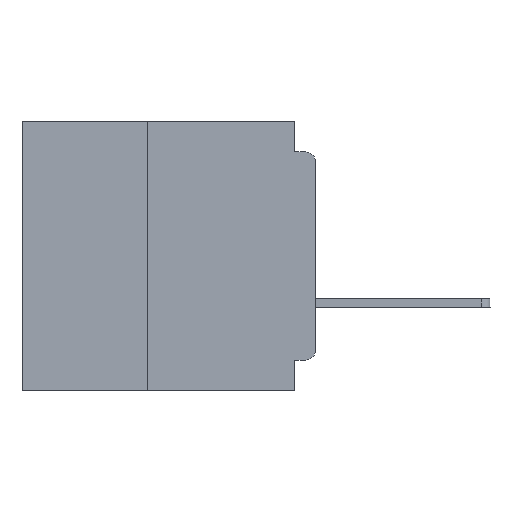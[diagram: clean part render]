
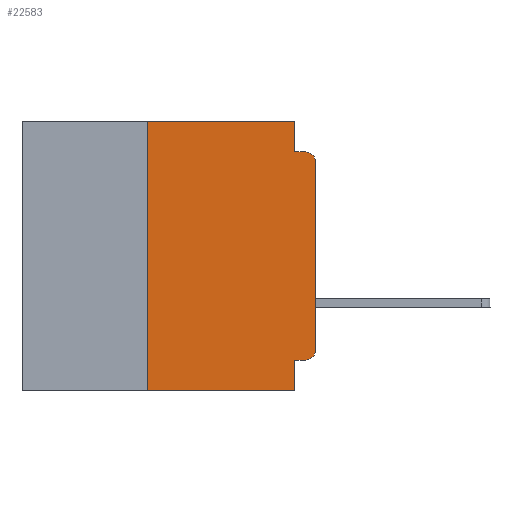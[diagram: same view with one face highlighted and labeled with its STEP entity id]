
A CAD part, left-side view. The second image highlights one B-rep face of the part: STEP entity #22583.
In plain terms, the highlighted planar face has unit normal (-1, 0, 0).
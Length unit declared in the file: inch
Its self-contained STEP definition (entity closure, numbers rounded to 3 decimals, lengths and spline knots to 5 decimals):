
#643 = ORIENTED_EDGE ( 'NONE', *, *, #54215, .T. ) ;
#1542 = DIRECTION ( 'NONE',  ( -1., 0., 0. ) ) ;
#1597 = ORIENTED_EDGE ( 'NONE', *, *, #41846, .F. ) ;
#3135 = VERTEX_POINT ( 'NONE', #16661 ) ;
#4061 = ORIENTED_EDGE ( 'NONE', *, *, #28307, .F. ) ;
#5367 = VECTOR ( 'NONE', #54887, 39.37008 ) ;
#5471 = VERTEX_POINT ( 'NONE', #65578 ) ;
#5751 = CARTESIAN_POINT ( 'NONE',  ( 0., 0.437, -0.4 ) ) ;
#8550 = EDGE_CURVE ( 'NONE', #5471, #65223, #45834, .T. ) ;
#8816 = LINE ( 'NONE', #59052, #59997 ) ;
#8886 = EDGE_CURVE ( 'NONE', #30488, #39142, #62537, .T. ) ;
#12045 = AXIS2_PLACEMENT_3D ( 'NONE', #50306, #45377, #14677 ) ;
#13266 = ORIENTED_EDGE ( 'NONE', *, *, #8550, .F. ) ;
#13970 = CARTESIAN_POINT ( 'NONE',  ( 0., 0.031, 0. ) ) ;
#14677 = DIRECTION ( 'NONE',  ( 0., 0., -1. ) ) ;
#14919 = FACE_OUTER_BOUND ( 'NONE', #15027, .T. ) ;
#15027 = EDGE_LOOP ( 'NONE', ( #643, #23600, #38655, #44543, #13266, #1597, #65956, #4061, #31773, #32027 ) ) ;
#16199 = CARTESIAN_POINT ( 'NONE',  ( 0., 0.015, -0.355 ) ) ;
#16441 = DIRECTION ( 'NONE',  ( -1., 0., 0. ) ) ;
#16661 = CARTESIAN_POINT ( 'NONE',  ( 0., 0.031, -0.4 ) ) ;
#18741 = AXIS2_PLACEMENT_3D ( 'NONE', #32315, #1542, #37465 ) ;
#18847 = AXIS2_PLACEMENT_3D ( 'NONE', #47138, #16441, #52256 ) ;
#20022 = CARTESIAN_POINT ( 'NONE',  ( 0., 0.25, -0.4 ) ) ;
#20144 = VECTOR ( 'NONE', #25814, 39.37008 ) ;
#20293 = CARTESIAN_POINT ( 'NONE',  ( 0., 0., 0. ) ) ;
#21737 = CARTESIAN_POINT ( 'NONE',  ( 0., 0.031, -0.045 ) ) ;
#22583 = ADVANCED_FACE ( 'NONE', ( #14919 ), #55152, .F. ) ;
#23600 = ORIENTED_EDGE ( 'NONE', *, *, #44344, .T. ) ;
#23817 = DIRECTION ( 'NONE',  ( 0., -1., 0. ) ) ;
#24776 = CARTESIAN_POINT ( 'NONE',  ( 0., 0., -0.355 ) ) ;
#25814 = DIRECTION ( 'NONE',  ( 0., 0., 1. ) ) ;
#28307 = EDGE_CURVE ( 'NONE', #39142, #3135, #32736, .T. ) ;
#30488 = VERTEX_POINT ( 'NONE', #16199 ) ;
#31773 = ORIENTED_EDGE ( 'NONE', *, *, #8886, .F. ) ;
#32027 = ORIENTED_EDGE ( 'NONE', *, *, #36684, .T. ) ;
#32076 = VECTOR ( 'NONE', #50921, 39.37008 ) ;
#32277 = EDGE_CURVE ( 'NONE', #51204, #55863, #8816, .T. ) ;
#32286 = VECTOR ( 'NONE', #57796, 39.37008 ) ;
#32315 = CARTESIAN_POINT ( 'NONE',  ( 0., 0.015, -0.06 ) ) ;
#32736 = LINE ( 'NONE', #62502, #58170 ) ;
#35287 = CARTESIAN_POINT ( 'NONE',  ( 0., 0.015, -0.045 ) ) ;
#36516 = LINE ( 'NONE', #5751, #63602 ) ;
#36539 = DIRECTION ( 'NONE',  ( 0., -1., 0. ) ) ;
#36684 = EDGE_CURVE ( 'NONE', #30488, #66147, #38762, .T. ) ;
#37465 = DIRECTION ( 'NONE',  ( 0., 0., -1. ) ) ;
#38655 = ORIENTED_EDGE ( 'NONE', *, *, #32277, .F. ) ;
#38762 = CIRCLE ( 'NONE', #18847, 0.015 ) ;
#39142 = VERTEX_POINT ( 'NONE', #43019 ) ;
#41498 = VERTEX_POINT ( 'NONE', #53520 ) ;
#41846 = EDGE_CURVE ( 'NONE', #47690, #5471, #45749, .T. ) ;
#43019 = CARTESIAN_POINT ( 'NONE',  ( 0., 0.031, -0.355 ) ) ;
#44344 = EDGE_CURVE ( 'NONE', #41498, #55863, #62130, .T. ) ;
#44543 = ORIENTED_EDGE ( 'NONE', *, *, #55248, .F. ) ;
#45377 = DIRECTION ( 'NONE',  ( 1., 0., 0. ) ) ;
#45749 = LINE ( 'NONE', #56334, #20144 ) ;
#45834 = LINE ( 'NONE', #47608, #32286 ) ;
#46270 = LINE ( 'NONE', #13970, #5367 ) ;
#47138 = CARTESIAN_POINT ( 'NONE',  ( 0., 0.015, -0.34 ) ) ;
#47608 = CARTESIAN_POINT ( 'NONE',  ( 0., 0.437, 0. ) ) ;
#47690 = VERTEX_POINT ( 'NONE', #20022 ) ;
#49012 = VECTOR ( 'NONE', #55296, 39.37008 ) ;
#50306 = CARTESIAN_POINT ( 'NONE',  ( 0., 0.437, 0. ) ) ;
#50921 = DIRECTION ( 'NONE',  ( 0., 0., 1. ) ) ;
#51204 = VERTEX_POINT ( 'NONE', #21737 ) ;
#52256 = DIRECTION ( 'NONE',  ( 0., 0., -1. ) ) ;
#53520 = CARTESIAN_POINT ( 'NONE',  ( 0., 0., -0.06 ) ) ;
#54215 = EDGE_CURVE ( 'NONE', #66147, #41498, #59141, .T. ) ;
#54887 = DIRECTION ( 'NONE',  ( 0., 0., -1. ) ) ;
#55152 = PLANE ( 'NONE',  #12045 ) ;
#55248 = EDGE_CURVE ( 'NONE', #65223, #51204, #46270, .T. ) ;
#55296 = DIRECTION ( 'NONE',  ( 0., 1., 0. ) ) ;
#55863 = VERTEX_POINT ( 'NONE', #35287 ) ;
#56334 = CARTESIAN_POINT ( 'NONE',  ( 0., 0.25, -0.4 ) ) ;
#56669 = EDGE_CURVE ( 'NONE', #47690, #3135, #36516, .T. ) ;
#57313 = DIRECTION ( 'NONE',  ( 0., 0., -1. ) ) ;
#57796 = DIRECTION ( 'NONE',  ( 0., -1., 0. ) ) ;
#58170 = VECTOR ( 'NONE', #57313, 39.37008 ) ;
#58590 = CARTESIAN_POINT ( 'NONE',  ( 0., 0., -0.34 ) ) ;
#59052 = CARTESIAN_POINT ( 'NONE',  ( 0., 0., -0.045 ) ) ;
#59141 = LINE ( 'NONE', #20293, #32076 ) ;
#59997 = VECTOR ( 'NONE', #23817, 39.37008 ) ;
#60621 = CARTESIAN_POINT ( 'NONE',  ( 0., 0.031, 0. ) ) ;
#62130 = CIRCLE ( 'NONE', #18741, 0.015 ) ;
#62502 = CARTESIAN_POINT ( 'NONE',  ( 0., 0.031, -0.4 ) ) ;
#62537 = LINE ( 'NONE', #24776, #49012 ) ;
#63602 = VECTOR ( 'NONE', #36539, 39.37008 ) ;
#65223 = VERTEX_POINT ( 'NONE', #60621 ) ;
#65578 = CARTESIAN_POINT ( 'NONE',  ( 0., 0.25, 0. ) ) ;
#65956 = ORIENTED_EDGE ( 'NONE', *, *, #56669, .T. ) ;
#66147 = VERTEX_POINT ( 'NONE', #58590 ) ;
